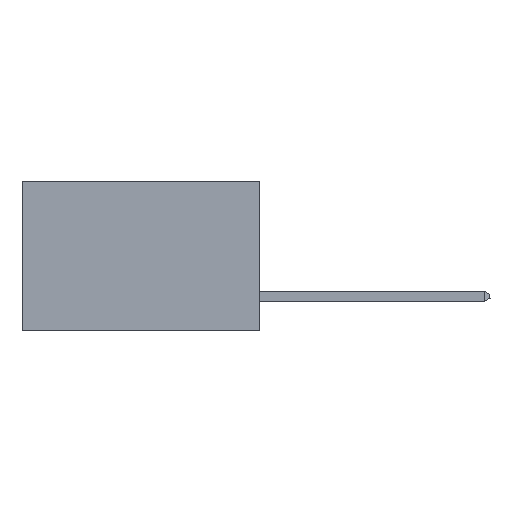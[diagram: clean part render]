
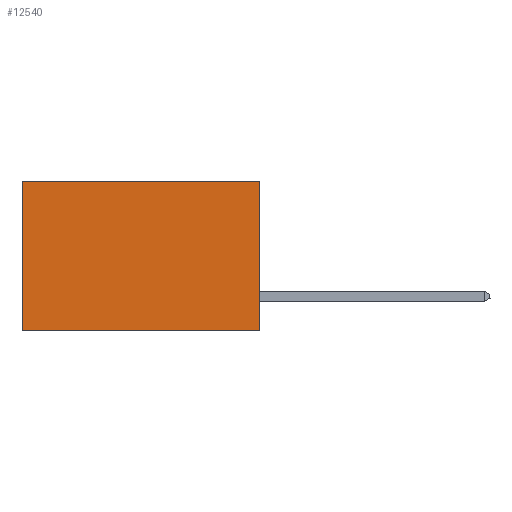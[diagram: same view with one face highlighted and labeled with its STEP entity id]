
A CAD part, left-side view. The second image highlights one B-rep face of the part: STEP entity #12540.
In plain terms, the highlighted planar face has unit normal (-1, 0, 0).
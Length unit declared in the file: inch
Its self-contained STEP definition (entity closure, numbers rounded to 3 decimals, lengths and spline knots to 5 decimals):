
#4 = DIRECTION ( 'NONE',  ( 0., 0., -1. ) ) ;
#532 = CARTESIAN_POINT ( 'NONE',  ( 0.277, 0.59, -0.37 ) ) ;
#1190 = CARTESIAN_POINT ( 'NONE',  ( 0.277, 0.59, -0.37 ) ) ;
#1947 = VECTOR ( 'NONE', #16347, 39.37008 ) ;
#2000 = EDGE_CURVE ( 'NONE', #16489, #10162, #2982, .T. ) ;
#2248 = EDGE_CURVE ( 'NONE', #15463, #16489, #12588, .T. ) ;
#2623 = CARTESIAN_POINT ( 'NONE',  ( 0.277, 0.59, 0. ) ) ;
#2665 = DIRECTION ( 'NONE',  ( 0., 1., 0. ) ) ;
#2982 = LINE ( 'NONE', #10184, #16601 ) ;
#3523 = LINE ( 'NONE', #532, #7119 ) ;
#4988 = DIRECTION ( 'NONE',  ( 1., 0., 0. ) ) ;
#6786 = DIRECTION ( 'NONE',  ( 0., 1., 0. ) ) ;
#7119 = VECTOR ( 'NONE', #4, 39.37008 ) ;
#7277 = ORIENTED_EDGE ( 'NONE', *, *, #2248, .F. ) ;
#7646 = CARTESIAN_POINT ( 'NONE',  ( 0.277, 0., -0.37 ) ) ;
#7738 = CARTESIAN_POINT ( 'NONE',  ( 0.277, 0., -0.37 ) ) ;
#7813 = ORIENTED_EDGE ( 'NONE', *, *, #9455, .T. ) ;
#8270 = EDGE_CURVE ( 'NONE', #15463, #16609, #8982, .T. ) ;
#8982 = LINE ( 'NONE', #9224, #9822 ) ;
#9208 = EDGE_LOOP ( 'NONE', ( #7813, #15668, #7277, #15944 ) ) ;
#9224 = CARTESIAN_POINT ( 'NONE',  ( 0.277, 0., 0. ) ) ;
#9455 = EDGE_CURVE ( 'NONE', #16609, #10162, #3523, .T. ) ;
#9822 = VECTOR ( 'NONE', #6786, 39.37008 ) ;
#10162 = VERTEX_POINT ( 'NONE', #1190 ) ;
#10184 = CARTESIAN_POINT ( 'NONE',  ( 0.277, 0., -0.37 ) ) ;
#10840 = AXIS2_PLACEMENT_3D ( 'NONE', #7646, #4988, #14331 ) ;
#10947 = CARTESIAN_POINT ( 'NONE',  ( 0.277, 0., 0. ) ) ;
#12540 = ADVANCED_FACE ( 'NONE', ( #16670 ), #13005, .F. ) ;
#12588 = LINE ( 'NONE', #15438, #1947 ) ;
#13005 = PLANE ( 'NONE',  #10840 ) ;
#14331 = DIRECTION ( 'NONE',  ( 0., 0., -1. ) ) ;
#15438 = CARTESIAN_POINT ( 'NONE',  ( 0.277, 0., -0.37 ) ) ;
#15463 = VERTEX_POINT ( 'NONE', #10947 ) ;
#15668 = ORIENTED_EDGE ( 'NONE', *, *, #2000, .F. ) ;
#15944 = ORIENTED_EDGE ( 'NONE', *, *, #8270, .T. ) ;
#16347 = DIRECTION ( 'NONE',  ( 0., 0., -1. ) ) ;
#16489 = VERTEX_POINT ( 'NONE', #7738 ) ;
#16601 = VECTOR ( 'NONE', #2665, 39.37008 ) ;
#16609 = VERTEX_POINT ( 'NONE', #2623 ) ;
#16670 = FACE_OUTER_BOUND ( 'NONE', #9208, .T. ) ;
